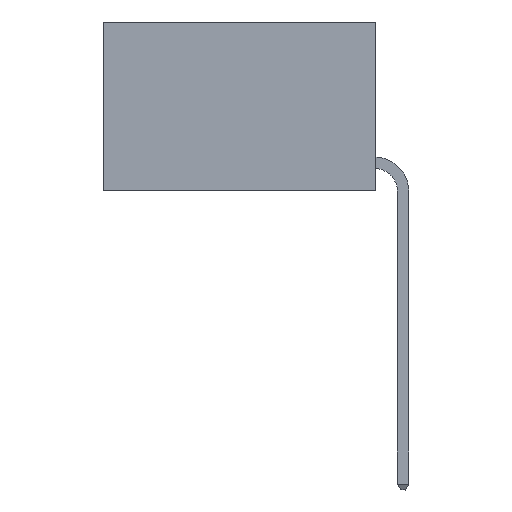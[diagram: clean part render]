
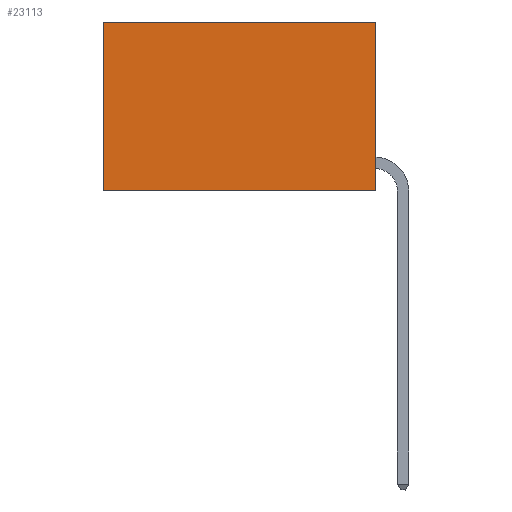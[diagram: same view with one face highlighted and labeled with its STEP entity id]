
A CAD part, left-side view. The second image highlights one B-rep face of the part: STEP entity #23113.
In plain terms, the highlighted planar face has unit normal (-1, 0, 0).
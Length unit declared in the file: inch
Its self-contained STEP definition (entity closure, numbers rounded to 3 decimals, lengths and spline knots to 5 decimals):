
#267 = VERTEX_POINT ( 'NONE', #15634 ) ;
#301 = ORIENTED_EDGE ( 'NONE', *, *, #5883, .F. ) ;
#311 = DIRECTION ( 'NONE',  ( 1., 0., 0. ) ) ;
#781 = ORIENTED_EDGE ( 'NONE', *, *, #19729, .T. ) ;
#1264 = VERTEX_POINT ( 'NONE', #2957 ) ;
#1589 = ORIENTED_EDGE ( 'NONE', *, *, #21931, .T. ) ;
#2116 = VECTOR ( 'NONE', #20413, 39.37008 ) ;
#2526 = VERTEX_POINT ( 'NONE', #12066 ) ;
#2716 = VECTOR ( 'NONE', #14936, 39.37008 ) ;
#2748 = LINE ( 'NONE', #4525, #2116 ) ;
#2957 = CARTESIAN_POINT ( 'NONE',  ( 0.2625, 0., -0.37 ) ) ;
#3832 = VECTOR ( 'NONE', #5332, 39.37008 ) ;
#4525 = CARTESIAN_POINT ( 'NONE',  ( 0.2625, 0., 0. ) ) ;
#5332 = DIRECTION ( 'NONE',  ( 0., 0., -1. ) ) ;
#5883 = EDGE_CURVE ( 'NONE', #267, #1264, #9225, .T. ) ;
#6159 = ORIENTED_EDGE ( 'NONE', *, *, #24833, .F. ) ;
#6945 = CARTESIAN_POINT ( 'NONE',  ( 0.2625, 0., -0.37 ) ) ;
#7288 = CARTESIAN_POINT ( 'NONE',  ( 0.2625, 0., 0. ) ) ;
#8093 = LINE ( 'NONE', #6945, #2716 ) ;
#9225 = LINE ( 'NONE', #7288, #3832 ) ;
#12066 = CARTESIAN_POINT ( 'NONE',  ( 0.2625, 0.6, -0.37 ) ) ;
#12338 = CARTESIAN_POINT ( 'NONE',  ( 0.2625, 0., 0. ) ) ;
#12692 = VERTEX_POINT ( 'NONE', #17051 ) ;
#14163 = AXIS2_PLACEMENT_3D ( 'NONE', #12338, #311, #14347 ) ;
#14347 = DIRECTION ( 'NONE',  ( 0., 0., -1. ) ) ;
#14936 = DIRECTION ( 'NONE',  ( 0., 1., 0. ) ) ;
#15634 = CARTESIAN_POINT ( 'NONE',  ( 0.2625, 0., 0. ) ) ;
#16084 = DIRECTION ( 'NONE',  ( 0., 0., -1. ) ) ;
#17051 = CARTESIAN_POINT ( 'NONE',  ( 0.2625, 0.6, 0. ) ) ;
#17861 = VECTOR ( 'NONE', #16084, 39.37008 ) ;
#18150 = FACE_OUTER_BOUND ( 'NONE', #18775, .T. ) ;
#18775 = EDGE_LOOP ( 'NONE', ( #781, #6159, #301, #1589 ) ) ;
#19729 = EDGE_CURVE ( 'NONE', #12692, #2526, #23116, .T. ) ;
#19914 = CARTESIAN_POINT ( 'NONE',  ( 0.2625, 0.6, 0. ) ) ;
#20413 = DIRECTION ( 'NONE',  ( 0., 1., 0. ) ) ;
#21931 = EDGE_CURVE ( 'NONE', #267, #12692, #2748, .T. ) ;
#23113 = ADVANCED_FACE ( 'NONE', ( #18150 ), #24228, .F. ) ;
#23116 = LINE ( 'NONE', #19914, #17861 ) ;
#24228 = PLANE ( 'NONE',  #14163 ) ;
#24833 = EDGE_CURVE ( 'NONE', #1264, #2526, #8093, .T. ) ;
